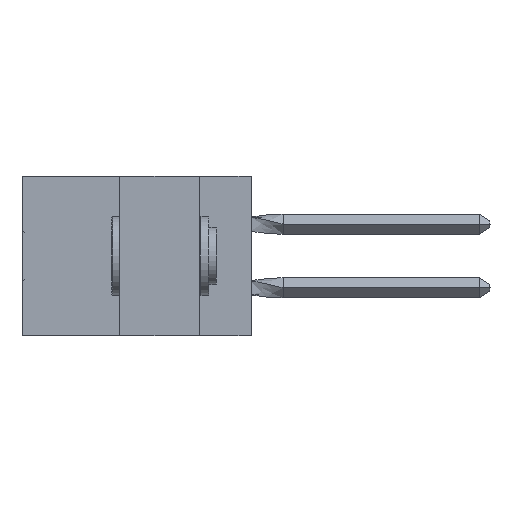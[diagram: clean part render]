
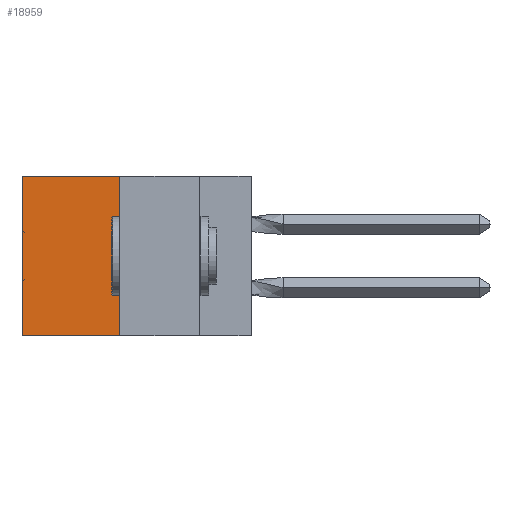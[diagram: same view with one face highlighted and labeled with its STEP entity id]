
A CAD part, left-side view. The second image highlights one B-rep face of the part: STEP entity #18959.
In plain terms, the highlighted planar face has unit normal (-1, 0, 0).
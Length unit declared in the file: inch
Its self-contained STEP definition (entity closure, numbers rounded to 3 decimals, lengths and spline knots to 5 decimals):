
#3685 = ORIENTED_EDGE ( 'NONE', *, *, #42963, .T. ) ;
#4012 = CARTESIAN_POINT ( 'NONE',  ( 0.305, 0.413, -0.5 ) ) ;
#5247 = CARTESIAN_POINT ( 'NONE',  ( 0.305, 0.72, -0.5 ) ) ;
#6252 = LINE ( 'NONE', #15823, #9177 ) ;
#8735 = DIRECTION ( 'NONE',  ( 0., 1., 0. ) ) ;
#9177 = VECTOR ( 'NONE', #8735, 39.37008 ) ;
#11030 = LINE ( 'NONE', #36247, #37561 ) ;
#11425 = CARTESIAN_POINT ( 'NONE',  ( 0.305, 0.413, 0. ) ) ;
#11513 = DIRECTION ( 'NONE',  ( 0., 0., -1. ) ) ;
#13170 = VERTEX_POINT ( 'NONE', #42387 ) ;
#14244 = DIRECTION ( 'NONE',  ( 0., 0., -1. ) ) ;
#15577 = FACE_OUTER_BOUND ( 'NONE', #42895, .T. ) ;
#15823 = CARTESIAN_POINT ( 'NONE',  ( 0.305, 0.413, -0.5 ) ) ;
#15829 = ORIENTED_EDGE ( 'NONE', *, *, #30301, .T. ) ;
#18959 = ADVANCED_FACE ( 'NONE', ( #15577 ), #40561, .F. ) ;
#23433 = EDGE_CURVE ( 'NONE', #37881, #37746, #28620, .T. ) ;
#25273 = CARTESIAN_POINT ( 'NONE',  ( 0.305, 0.413, -0.5 ) ) ;
#26297 = VECTOR ( 'NONE', #43395, 39.37008 ) ;
#28620 = LINE ( 'NONE', #4012, #42737 ) ;
#28951 = DIRECTION ( 'NONE',  ( 0., 1., 0. ) ) ;
#29649 = CARTESIAN_POINT ( 'NONE',  ( 0.305, 0.72, 0. ) ) ;
#30301 = EDGE_CURVE ( 'NONE', #35594, #13170, #46304, .T. ) ;
#31088 = ORIENTED_EDGE ( 'NONE', *, *, #35740, .F. ) ;
#33525 = CARTESIAN_POINT ( 'NONE',  ( 0.305, 0.413, -0.5 ) ) ;
#35594 = VERTEX_POINT ( 'NONE', #29649 ) ;
#35740 = EDGE_CURVE ( 'NONE', #37746, #13170, #6252, .T. ) ;
#36247 = CARTESIAN_POINT ( 'NONE',  ( 0.305, 0.413, 0. ) ) ;
#37561 = VECTOR ( 'NONE', #28951, 39.37008 ) ;
#37746 = VERTEX_POINT ( 'NONE', #33525 ) ;
#37881 = VERTEX_POINT ( 'NONE', #11425 ) ;
#40561 = PLANE ( 'NONE',  #44122 ) ;
#42387 = CARTESIAN_POINT ( 'NONE',  ( 0.305, 0.72, -0.5 ) ) ;
#42737 = VECTOR ( 'NONE', #11513, 39.37008 ) ;
#42895 = EDGE_LOOP ( 'NONE', ( #15829, #31088, #46788, #3685 ) ) ;
#42963 = EDGE_CURVE ( 'NONE', #37881, #35594, #11030, .T. ) ;
#43395 = DIRECTION ( 'NONE',  ( 0., 0., -1. ) ) ;
#44122 = AXIS2_PLACEMENT_3D ( 'NONE', #25273, #44198, #14244 ) ;
#44198 = DIRECTION ( 'NONE',  ( 1., 0., 0. ) ) ;
#46304 = LINE ( 'NONE', #5247, #26297 ) ;
#46788 = ORIENTED_EDGE ( 'NONE', *, *, #23433, .F. ) ;
